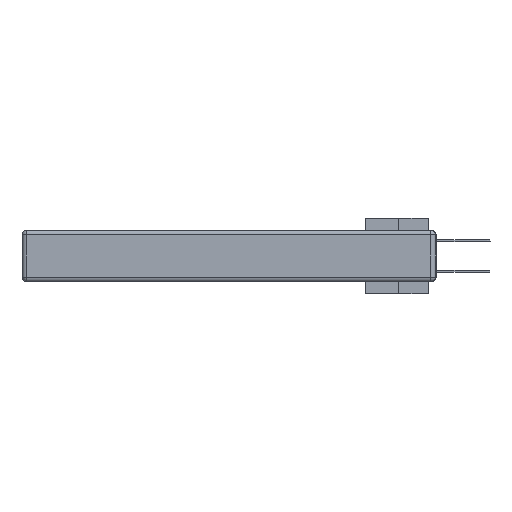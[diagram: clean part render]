
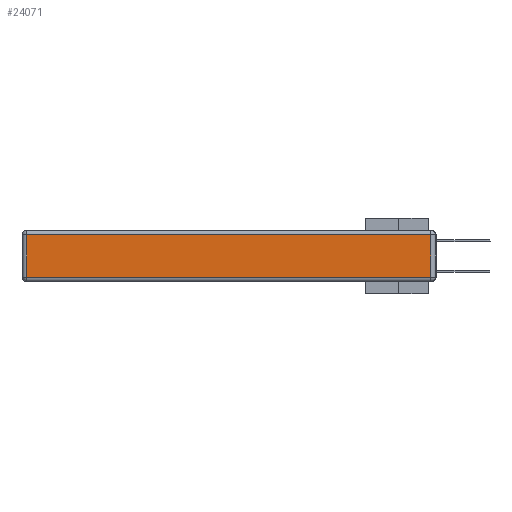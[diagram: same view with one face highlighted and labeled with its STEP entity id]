
A CAD part, left-side view. The second image highlights one B-rep face of the part: STEP entity #24071.
In plain terms, the highlighted planar face has unit normal (-1, 0, 0).
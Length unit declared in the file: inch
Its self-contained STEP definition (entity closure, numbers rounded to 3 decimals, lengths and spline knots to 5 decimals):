
#470 = LINE ( 'NONE', #6023, #29625 ) ;
#523 = EDGE_CURVE ( 'NONE', #12261, #37629, #470, .T. ) ;
#613 = EDGE_CURVE ( 'NONE', #24086, #2970, #24605, .T. ) ;
#1655 = CARTESIAN_POINT ( 'NONE',  ( 0., 0.03, -0.03 ) ) ;
#2970 = VERTEX_POINT ( 'NONE', #8795 ) ;
#4005 = EDGE_LOOP ( 'NONE', ( #6860, #27380, #12539, #30734 ) ) ;
#6023 = CARTESIAN_POINT ( 'NONE',  ( 0., 2.75, -0.03 ) ) ;
#6764 = DIRECTION ( 'NONE',  ( 0., -1., 0. ) ) ;
#6860 = ORIENTED_EDGE ( 'NONE', *, *, #613, .T. ) ;
#7882 = DIRECTION ( 'NONE',  ( -1., 0., 0. ) ) ;
#8092 = FACE_OUTER_BOUND ( 'NONE', #4005, .T. ) ;
#8140 = CARTESIAN_POINT ( 'NONE',  ( 0., 2.72, -0.313 ) ) ;
#8761 = VECTOR ( 'NONE', #6764, 39.37008 ) ;
#8795 = CARTESIAN_POINT ( 'NONE',  ( 0., 0.03, -0.313 ) ) ;
#9868 = CARTESIAN_POINT ( 'NONE',  ( 0., 0., -0.313 ) ) ;
#10601 = CARTESIAN_POINT ( 'NONE',  ( 0., 0., -0.343 ) ) ;
#12261 = VERTEX_POINT ( 'NONE', #1655 ) ;
#12539 = ORIENTED_EDGE ( 'NONE', *, *, #523, .T. ) ;
#13139 = EDGE_CURVE ( 'NONE', #37629, #24086, #18485, .T. ) ;
#13479 = DIRECTION ( 'NONE',  ( 0., 0., 1. ) ) ;
#13959 = PLANE ( 'NONE',  #27028 ) ;
#15147 = DIRECTION ( 'NONE',  ( 0., 0., 1. ) ) ;
#16390 = CARTESIAN_POINT ( 'NONE',  ( 0., 2.72, -0.03 ) ) ;
#16751 = CARTESIAN_POINT ( 'NONE',  ( 0., 2.72, -0.343 ) ) ;
#16923 = LINE ( 'NONE', #26950, #21486 ) ;
#18485 = LINE ( 'NONE', #16751, #29404 ) ;
#20624 = DIRECTION ( 'NONE',  ( 0., 1., 0. ) ) ;
#21486 = VECTOR ( 'NONE', #15147, 39.37008 ) ;
#23497 = DIRECTION ( 'NONE',  ( 0., 0., -1. ) ) ;
#24071 = ADVANCED_FACE ( 'NONE', ( #8092 ), #13959, .T. ) ;
#24086 = VERTEX_POINT ( 'NONE', #8140 ) ;
#24605 = LINE ( 'NONE', #9868, #8761 ) ;
#26950 = CARTESIAN_POINT ( 'NONE',  ( 0., 0.03, -0.343 ) ) ;
#27028 = AXIS2_PLACEMENT_3D ( 'NONE', #10601, #7882, #13479 ) ;
#27380 = ORIENTED_EDGE ( 'NONE', *, *, #37486, .T. ) ;
#29404 = VECTOR ( 'NONE', #23497, 39.37008 ) ;
#29625 = VECTOR ( 'NONE', #20624, 39.37008 ) ;
#30734 = ORIENTED_EDGE ( 'NONE', *, *, #13139, .T. ) ;
#37486 = EDGE_CURVE ( 'NONE', #2970, #12261, #16923, .T. ) ;
#37629 = VERTEX_POINT ( 'NONE', #16390 ) ;
